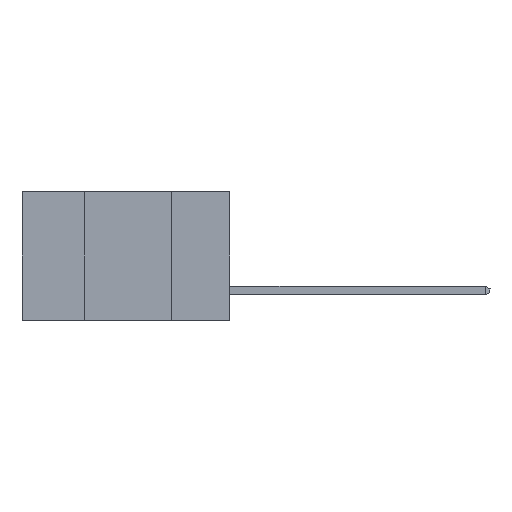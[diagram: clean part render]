
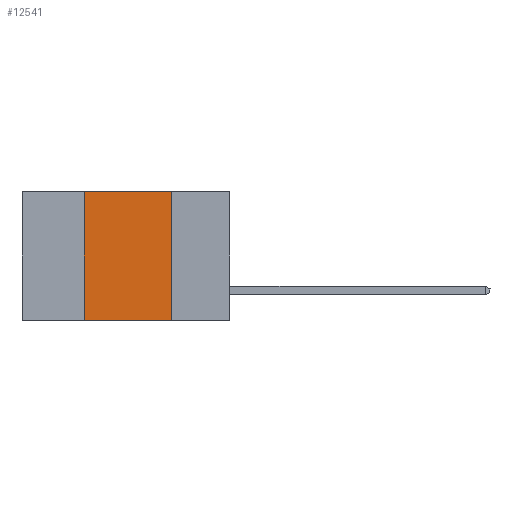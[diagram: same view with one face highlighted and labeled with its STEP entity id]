
A CAD part, left-side view. The second image highlights one B-rep face of the part: STEP entity #12541.
In plain terms, the highlighted planar face has unit normal (-1, 0, 0).
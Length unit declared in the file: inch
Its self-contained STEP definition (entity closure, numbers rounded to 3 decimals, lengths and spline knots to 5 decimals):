
#243 = DIRECTION ( 'NONE',  ( 0., 0., 1. ) ) ;
#245 = ORIENTED_EDGE ( 'NONE', *, *, #9554, .F. ) ;
#620 = CARTESIAN_POINT ( 'NONE',  ( 0., 0.6, 0. ) ) ;
#950 = VECTOR ( 'NONE', #11137, 39.37008 ) ;
#969 = CARTESIAN_POINT ( 'NONE',  ( 0., 0.42, -0.37 ) ) ;
#1357 = EDGE_CURVE ( 'NONE', #3917, #14331, #5946, .T. ) ;
#1768 = LINE ( 'NONE', #620, #3628 ) ;
#2097 = FACE_OUTER_BOUND ( 'NONE', #11997, .T. ) ;
#2125 = DIRECTION ( 'NONE',  ( 0., 0., -1. ) ) ;
#3628 = VECTOR ( 'NONE', #4573, 39.37008 ) ;
#3917 = VERTEX_POINT ( 'NONE', #969 ) ;
#4013 = VERTEX_POINT ( 'NONE', #13750 ) ;
#4573 = DIRECTION ( 'NONE',  ( 0., -1., 0. ) ) ;
#5204 = CARTESIAN_POINT ( 'NONE',  ( 0., 0.6, -0.37 ) ) ;
#5522 = PLANE ( 'NONE',  #10948 ) ;
#5565 = CARTESIAN_POINT ( 'NONE',  ( 0., 0.17, -0.37 ) ) ;
#5600 = DIRECTION ( 'NONE',  ( 1., 0., 0. ) ) ;
#5946 = LINE ( 'NONE', #10668, #6445 ) ;
#6445 = VECTOR ( 'NONE', #243, 39.37008 ) ;
#7799 = LINE ( 'NONE', #5204, #950 ) ;
#8178 = ORIENTED_EDGE ( 'NONE', *, *, #11612, .T. ) ;
#8943 = DIRECTION ( 'NONE',  ( 0., 0., -1. ) ) ;
#9554 = EDGE_CURVE ( 'NONE', #14331, #4013, #1768, .T. ) ;
#9611 = VERTEX_POINT ( 'NONE', #5565 ) ;
#10379 = EDGE_CURVE ( 'NONE', #4013, #9611, #14481, .T. ) ;
#10668 = CARTESIAN_POINT ( 'NONE',  ( 0., 0.42, -0.37 ) ) ;
#10893 = VECTOR ( 'NONE', #2125, 39.37008 ) ;
#10948 = AXIS2_PLACEMENT_3D ( 'NONE', #12227, #5600, #8943 ) ;
#11137 = DIRECTION ( 'NONE',  ( 0., -1., 0. ) ) ;
#11235 = CARTESIAN_POINT ( 'NONE',  ( 0., 0.42, 0. ) ) ;
#11612 = EDGE_CURVE ( 'NONE', #3917, #9611, #7799, .T. ) ;
#11997 = EDGE_LOOP ( 'NONE', ( #13565, #245, #13096, #8178 ) ) ;
#12227 = CARTESIAN_POINT ( 'NONE',  ( 0., 0.6, 0. ) ) ;
#12541 = ADVANCED_FACE ( 'NONE', ( #2097 ), #5522, .F. ) ;
#13096 = ORIENTED_EDGE ( 'NONE', *, *, #1357, .F. ) ;
#13565 = ORIENTED_EDGE ( 'NONE', *, *, #10379, .F. ) ;
#13690 = CARTESIAN_POINT ( 'NONE',  ( 0., 0.17, -0.37 ) ) ;
#13750 = CARTESIAN_POINT ( 'NONE',  ( 0., 0.17, 0. ) ) ;
#14331 = VERTEX_POINT ( 'NONE', #11235 ) ;
#14481 = LINE ( 'NONE', #13690, #10893 ) ;
